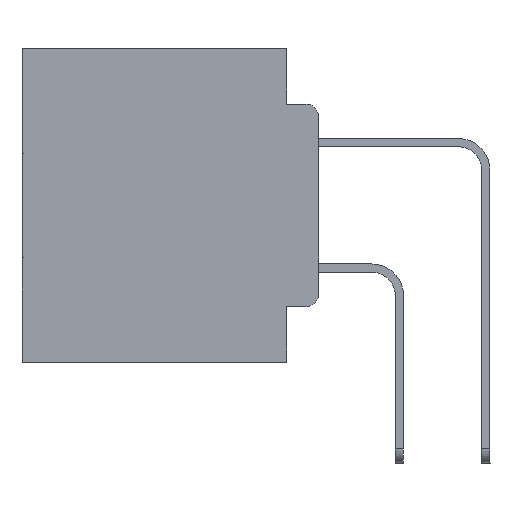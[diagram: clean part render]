
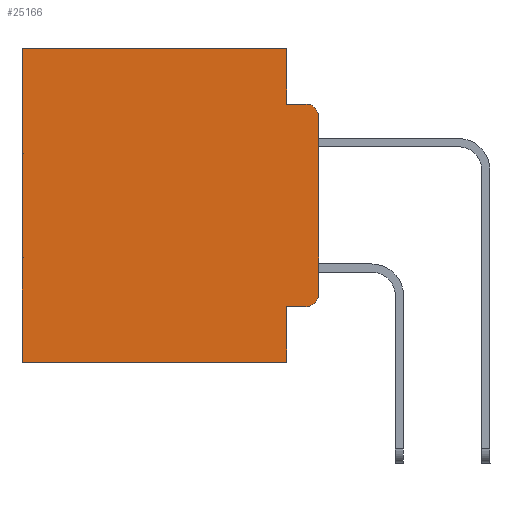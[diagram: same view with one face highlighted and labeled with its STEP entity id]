
A CAD part, left-side view. The second image highlights one B-rep face of the part: STEP entity #25166.
In plain terms, the highlighted planar face has unit normal (-1, 0, 0).
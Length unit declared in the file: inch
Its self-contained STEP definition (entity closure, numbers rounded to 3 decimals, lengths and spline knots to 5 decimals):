
#228 = DIRECTION ( 'NONE',  ( 0., -1., 0. ) ) ;
#433 = CARTESIAN_POINT ( 'NONE',  ( 0.298, 0.02, -0.4115 ) ) ;
#1035 = DIRECTION ( 'NONE',  ( -1., 0., 0. ) ) ;
#1229 = ORIENTED_EDGE ( 'NONE', *, *, #18729, .T. ) ;
#1610 = CARTESIAN_POINT ( 'NONE',  ( 0.298, 0.473, 0. ) ) ;
#1676 = CARTESIAN_POINT ( 'NONE',  ( 0.298, 0.02, -0.0885 ) ) ;
#2228 = CARTESIAN_POINT ( 'NONE',  ( 0.298, 0., -0.5 ) ) ;
#2314 = VERTEX_POINT ( 'NONE', #1676 ) ;
#2803 = VECTOR ( 'NONE', #18904, 39.37008 ) ;
#3643 = LINE ( 'NONE', #6234, #2803 ) ;
#3975 = VERTEX_POINT ( 'NONE', #30027 ) ;
#3979 = LINE ( 'NONE', #32722, #14477 ) ;
#4130 = ORIENTED_EDGE ( 'NONE', *, *, #25399, .T. ) ;
#4133 = CARTESIAN_POINT ( 'NONE',  ( 0.298, 0.051, -0.4115 ) ) ;
#4732 = DIRECTION ( 'NONE',  ( 0., 1., 0. ) ) ;
#4998 = AXIS2_PLACEMENT_3D ( 'NONE', #8528, #11134, #28578 ) ;
#5507 = EDGE_CURVE ( 'NONE', #17885, #18479, #25014, .T. ) ;
#5573 = CARTESIAN_POINT ( 'NONE',  ( 0.298, 0.051, -0.0885 ) ) ;
#6234 = CARTESIAN_POINT ( 'NONE',  ( 0.298, 0.051, 0. ) ) ;
#7123 = DIRECTION ( 'NONE',  ( 0., 0., -1. ) ) ;
#7427 = VECTOR ( 'NONE', #27080, 39.37008 ) ;
#8250 = ORIENTED_EDGE ( 'NONE', *, *, #11599, .T. ) ;
#8528 = CARTESIAN_POINT ( 'NONE',  ( 0.298, 0., 0. ) ) ;
#8550 = EDGE_CURVE ( 'NONE', #15235, #28818, #27876, .T. ) ;
#9283 = CARTESIAN_POINT ( 'NONE',  ( 0.298, 0.051, -0.0885 ) ) ;
#9379 = VERTEX_POINT ( 'NONE', #4133 ) ;
#9880 = CARTESIAN_POINT ( 'NONE',  ( 0.298, 0., 0. ) ) ;
#10302 = EDGE_CURVE ( 'NONE', #9379, #15235, #3979, .T. ) ;
#11134 = DIRECTION ( 'NONE',  ( 1., 0., 0. ) ) ;
#11143 = LINE ( 'NONE', #5573, #27923 ) ;
#11205 = CARTESIAN_POINT ( 'NONE',  ( 0.298, 0.051, -0.5 ) ) ;
#11599 = EDGE_CURVE ( 'NONE', #3975, #14406, #15962, .T. ) ;
#12113 = DIRECTION ( 'NONE',  ( -1., 0., 0. ) ) ;
#13051 = CIRCLE ( 'NONE', #28645, 0.02 ) ;
#14232 = LINE ( 'NONE', #1610, #7427 ) ;
#14406 = VERTEX_POINT ( 'NONE', #20179 ) ;
#14477 = VECTOR ( 'NONE', #15439, 39.37008 ) ;
#15175 = VECTOR ( 'NONE', #4732, 39.37008 ) ;
#15235 = VERTEX_POINT ( 'NONE', #433 ) ;
#15359 = EDGE_CURVE ( 'NONE', #9379, #17885, #3643, .T. ) ;
#15399 = ORIENTED_EDGE ( 'NONE', *, *, #28702, .F. ) ;
#15439 = DIRECTION ( 'NONE',  ( 0., -1., 0. ) ) ;
#15764 = VERTEX_POINT ( 'NONE', #17903 ) ;
#15818 = ORIENTED_EDGE ( 'NONE', *, *, #5507, .F. ) ;
#15962 = LINE ( 'NONE', #9880, #15175 ) ;
#16087 = AXIS2_PLACEMENT_3D ( 'NONE', #16530, #1035, #19054 ) ;
#16530 = CARTESIAN_POINT ( 'NONE',  ( 0.298, 0.02, -0.3915 ) ) ;
#16963 = ORIENTED_EDGE ( 'NONE', *, *, #23735, .F. ) ;
#17885 = VERTEX_POINT ( 'NONE', #11205 ) ;
#17903 = CARTESIAN_POINT ( 'NONE',  ( 0.298, 0., -0.1085 ) ) ;
#18394 = VECTOR ( 'NONE', #27665, 39.37008 ) ;
#18479 = VERTEX_POINT ( 'NONE', #26030 ) ;
#18729 = EDGE_CURVE ( 'NONE', #14406, #18479, #14232, .T. ) ;
#18904 = DIRECTION ( 'NONE',  ( 0., 0., -1. ) ) ;
#19054 = DIRECTION ( 'NONE',  ( 0., 0., -1. ) ) ;
#19333 = ORIENTED_EDGE ( 'NONE', *, *, #20401, .F. ) ;
#19760 = CARTESIAN_POINT ( 'NONE',  ( 0.298, 0., 0. ) ) ;
#20179 = CARTESIAN_POINT ( 'NONE',  ( 0.298, 0.473, 0. ) ) ;
#20401 = EDGE_CURVE ( 'NONE', #3975, #28637, #25425, .T. ) ;
#22473 = ORIENTED_EDGE ( 'NONE', *, *, #10302, .T. ) ;
#23609 = PLANE ( 'NONE',  #4998 ) ;
#23735 = EDGE_CURVE ( 'NONE', #28637, #2314, #11143, .T. ) ;
#24028 = ORIENTED_EDGE ( 'NONE', *, *, #8550, .T. ) ;
#24919 = LINE ( 'NONE', #19760, #30704 ) ;
#25014 = LINE ( 'NONE', #2228, #18394 ) ;
#25069 = CARTESIAN_POINT ( 'NONE',  ( 0.298, 0., -0.3915 ) ) ;
#25166 = ADVANCED_FACE ( 'NONE', ( #32438 ), #23609, .F. ) ;
#25399 = EDGE_CURVE ( 'NONE', #15764, #2314, #13051, .T. ) ;
#25425 = LINE ( 'NONE', #26734, #30427 ) ;
#26030 = CARTESIAN_POINT ( 'NONE',  ( 0.298, 0.473, -0.5 ) ) ;
#26734 = CARTESIAN_POINT ( 'NONE',  ( 0.298, 0.051, 0. ) ) ;
#27046 = CARTESIAN_POINT ( 'NONE',  ( 0.298, 0.02, -0.1085 ) ) ;
#27080 = DIRECTION ( 'NONE',  ( 0., 0., -1. ) ) ;
#27665 = DIRECTION ( 'NONE',  ( 0., 1., 0. ) ) ;
#27876 = CIRCLE ( 'NONE', #16087, 0.02 ) ;
#27923 = VECTOR ( 'NONE', #228, 39.37008 ) ;
#28578 = DIRECTION ( 'NONE',  ( 0., 0., -1. ) ) ;
#28637 = VERTEX_POINT ( 'NONE', #9283 ) ;
#28645 = AXIS2_PLACEMENT_3D ( 'NONE', #27046, #12113, #29527 ) ;
#28702 = EDGE_CURVE ( 'NONE', #15764, #28818, #24919, .T. ) ;
#28818 = VERTEX_POINT ( 'NONE', #25069 ) ;
#29032 = ORIENTED_EDGE ( 'NONE', *, *, #15359, .F. ) ;
#29216 = DIRECTION ( 'NONE',  ( 0., 0., -1. ) ) ;
#29527 = DIRECTION ( 'NONE',  ( 0., 0., -1. ) ) ;
#30027 = CARTESIAN_POINT ( 'NONE',  ( 0.298, 0.051, 0. ) ) ;
#30427 = VECTOR ( 'NONE', #29216, 39.37008 ) ;
#30704 = VECTOR ( 'NONE', #7123, 39.37008 ) ;
#31589 = EDGE_LOOP ( 'NONE', ( #15399, #4130, #16963, #19333, #8250, #1229, #15818, #29032, #22473, #24028 ) ) ;
#32438 = FACE_OUTER_BOUND ( 'NONE', #31589, .T. ) ;
#32722 = CARTESIAN_POINT ( 'NONE',  ( 0.298, 0.051, -0.4115 ) ) ;
